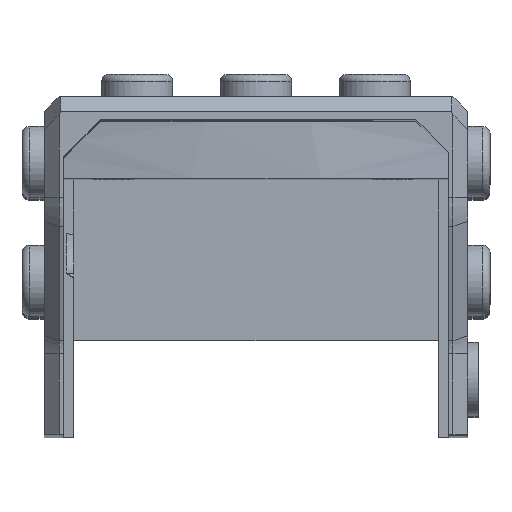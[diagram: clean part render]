
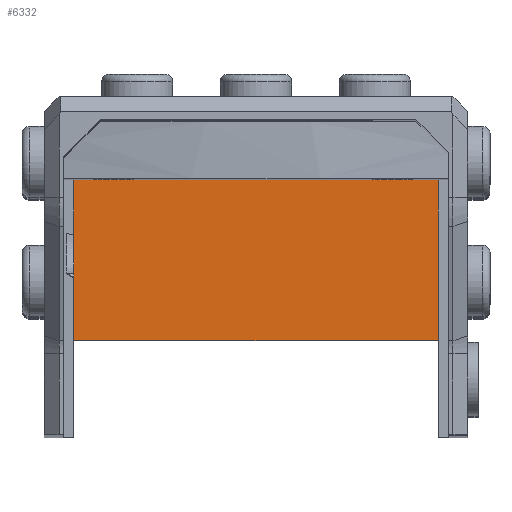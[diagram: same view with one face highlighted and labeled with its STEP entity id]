
A CAD part, top view. The second image highlights one B-rep face of the part: STEP entity #6332.
In plain terms, the highlighted planar face has unit normal (0, 0, 1).
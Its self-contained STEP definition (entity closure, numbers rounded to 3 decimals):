
#547=ORIENTED_EDGE('',*,*,#2195,.F.);
#548=ORIENTED_EDGE('',*,*,#2196,.T.);
#549=ORIENTED_EDGE('',*,*,#2197,.F.);
#550=ORIENTED_EDGE('',*,*,#2198,.F.);
#551=ORIENTED_EDGE('',*,*,#2199,.F.);
#552=ORIENTED_EDGE('',*,*,#2200,.F.);
#2195=EDGE_CURVE('',#3019,#3020,#3648,.T.);
#2196=EDGE_CURVE('',#3019,#3021,#3649,.T.);
#2197=EDGE_CURVE('',#3022,#3021,#3650,.T.);
#2198=EDGE_CURVE('',#3023,#3022,#3651,.T.);
#2199=EDGE_CURVE('',#3024,#3023,#3652,.T.);
#2200=EDGE_CURVE('',#3020,#3024,#3653,.T.);
#3019=VERTEX_POINT('',#9433);
#3020=VERTEX_POINT('',#9434);
#3021=VERTEX_POINT('',#9436);
#3022=VERTEX_POINT('',#9438);
#3023=VERTEX_POINT('',#9440);
#3024=VERTEX_POINT('',#9442);
#3648=LINE('',#9432,#4147);
#3649=LINE('',#9435,#4148);
#3650=LINE('',#9437,#4149);
#3651=LINE('',#9439,#4150);
#3652=LINE('',#9441,#4151);
#3653=LINE('',#9443,#4152);
#4147=VECTOR('',#7519,1000.);
#4148=VECTOR('',#7520,1000.);
#4149=VECTOR('',#7521,1000.);
#4150=VECTOR('',#7522,1000.);
#4151=VECTOR('',#7523,1000.);
#4152=VECTOR('',#7524,1000.);
#4646=EDGE_LOOP('',(#547,#548,#549,#550,#551,#552));
#5363=FACE_BOUND('',#4646,.T.);
#6080=PLANE('',#6808);
#6332=ADVANCED_FACE('',(#5363),#6080,.T.);
#6808=AXIS2_PLACEMENT_3D('',#9431,#7517,#7518);
#7517=DIRECTION('',(0.,0.,1.));
#7518=DIRECTION('',(1.,0.,0.));
#7519=DIRECTION('',(0.,1.,0.));
#7520=DIRECTION('',(1.,0.,0.));
#7521=DIRECTION('',(0.,-1.,0.));
#7522=DIRECTION('',(0.707,-0.707,0.));
#7523=DIRECTION('',(1.,0.,0.));
#7524=DIRECTION('',(0.707,0.707,0.));
#9431=CARTESIAN_POINT('',(0.,0.,-1.));
#9432=CARTESIAN_POINT('',(-12.268,0.254,-1.));
#9433=CARTESIAN_POINT('',(-12.268,6.782,-1.));
#9434=CARTESIAN_POINT('',(-12.268,18.967,-1.));
#9435=CARTESIAN_POINT('',(0.,6.782,-1.));
#9436=CARTESIAN_POINT('',(12.268,6.782,-1.));
#9437=CARTESIAN_POINT('',(12.268,0.254,-1.));
#9438=CARTESIAN_POINT('',(12.268,18.967,-1.));
#9439=CARTESIAN_POINT('',(9.772,21.463,-1.));
#9440=CARTESIAN_POINT('',(9.772,21.463,-1.));
#9441=CARTESIAN_POINT('',(9.772,21.463,-1.));
#9442=CARTESIAN_POINT('',(-9.772,21.463,-1.));
#9443=CARTESIAN_POINT('',(-9.772,21.463,-1.));
